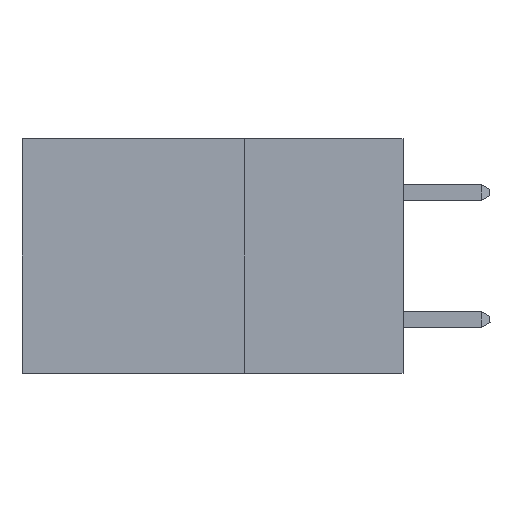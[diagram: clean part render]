
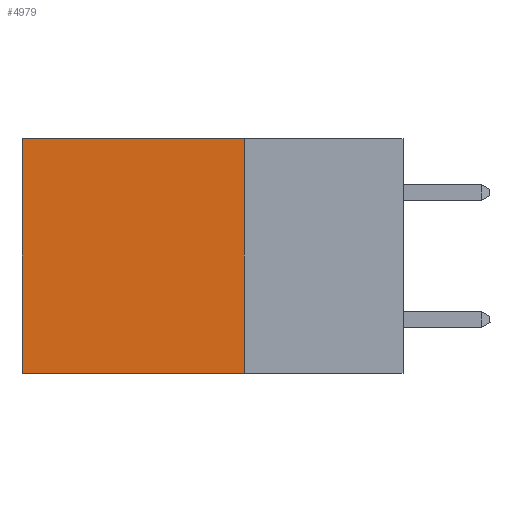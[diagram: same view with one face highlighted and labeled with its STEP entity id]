
A CAD part, left-side view. The second image highlights one B-rep face of the part: STEP entity #4979.
In plain terms, the highlighted planar face has unit normal (-1, 0, 0).
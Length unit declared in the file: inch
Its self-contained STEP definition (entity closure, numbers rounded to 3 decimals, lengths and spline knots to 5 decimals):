
#200 = DIRECTION ( 'NONE',  ( 0., 0., -1. ) ) ;
#814 = CARTESIAN_POINT ( 'NONE',  ( 0.2875, 0.25, 0. ) ) ;
#972 = FACE_OUTER_BOUND ( 'NONE', #2174, .T. ) ;
#1070 = DIRECTION ( 'NONE',  ( 0., 1., 0. ) ) ;
#1782 = ORIENTED_EDGE ( 'NONE', *, *, #2210, .F. ) ;
#2174 = EDGE_LOOP ( 'NONE', ( #14762, #7167, #1782, #16157 ) ) ;
#2210 = EDGE_CURVE ( 'NONE', #11049, #13108, #12747, .T. ) ;
#2459 = DIRECTION ( 'NONE',  ( 0., 0., -1. ) ) ;
#2985 = LINE ( 'NONE', #8013, #20834 ) ;
#4650 = DIRECTION ( 'NONE',  ( 0., 0., -1. ) ) ;
#4926 = VERTEX_POINT ( 'NONE', #12589 ) ;
#4979 = ADVANCED_FACE ( 'NONE', ( #972 ), #20904, .F. ) ;
#5067 = LINE ( 'NONE', #19665, #18429 ) ;
#7167 = ORIENTED_EDGE ( 'NONE', *, *, #13065, .F. ) ;
#7304 = LINE ( 'NONE', #814, #20142 ) ;
#8013 = CARTESIAN_POINT ( 'NONE',  ( 0.2875, 0.6, 0. ) ) ;
#10993 = CARTESIAN_POINT ( 'NONE',  ( 0.2875, 0.25, 0. ) ) ;
#11049 = VERTEX_POINT ( 'NONE', #14202 ) ;
#11074 = DIRECTION ( 'NONE',  ( 0., 1., 0. ) ) ;
#12234 = VECTOR ( 'NONE', #200, 39.37008 ) ;
#12589 = CARTESIAN_POINT ( 'NONE',  ( 0.2875, 0.6, 0. ) ) ;
#12659 = DIRECTION ( 'NONE',  ( 1., 0., 0. ) ) ;
#12747 = LINE ( 'NONE', #13767, #12234 ) ;
#13065 = EDGE_CURVE ( 'NONE', #13108, #16075, #5067, .T. ) ;
#13108 = VERTEX_POINT ( 'NONE', #13233 ) ;
#13233 = CARTESIAN_POINT ( 'NONE',  ( 0.2875, 0.25, -0.37 ) ) ;
#13767 = CARTESIAN_POINT ( 'NONE',  ( 0.2875, 0.25, 0. ) ) ;
#14130 = AXIS2_PLACEMENT_3D ( 'NONE', #10993, #12659, #2459 ) ;
#14202 = CARTESIAN_POINT ( 'NONE',  ( 0.2875, 0.25, 0. ) ) ;
#14762 = ORIENTED_EDGE ( 'NONE', *, *, #21535, .T. ) ;
#16075 = VERTEX_POINT ( 'NONE', #20584 ) ;
#16157 = ORIENTED_EDGE ( 'NONE', *, *, #20139, .T. ) ;
#18429 = VECTOR ( 'NONE', #1070, 39.37008 ) ;
#19665 = CARTESIAN_POINT ( 'NONE',  ( 0.2875, 0.25, -0.37 ) ) ;
#20139 = EDGE_CURVE ( 'NONE', #11049, #4926, #7304, .T. ) ;
#20142 = VECTOR ( 'NONE', #11074, 39.37008 ) ;
#20584 = CARTESIAN_POINT ( 'NONE',  ( 0.2875, 0.6, -0.37 ) ) ;
#20834 = VECTOR ( 'NONE', #4650, 39.37008 ) ;
#20904 = PLANE ( 'NONE',  #14130 ) ;
#21535 = EDGE_CURVE ( 'NONE', #4926, #16075, #2985, .T. ) ;
